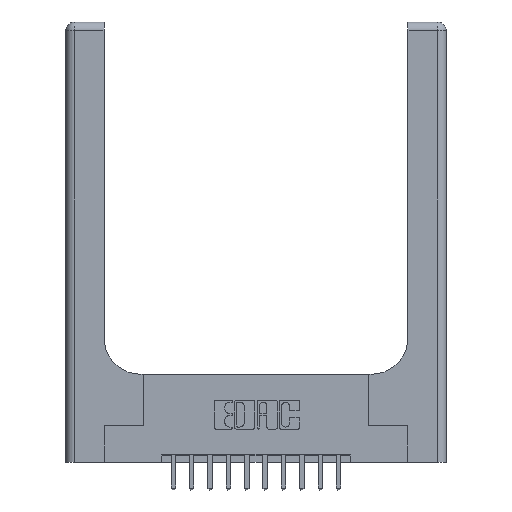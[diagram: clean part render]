
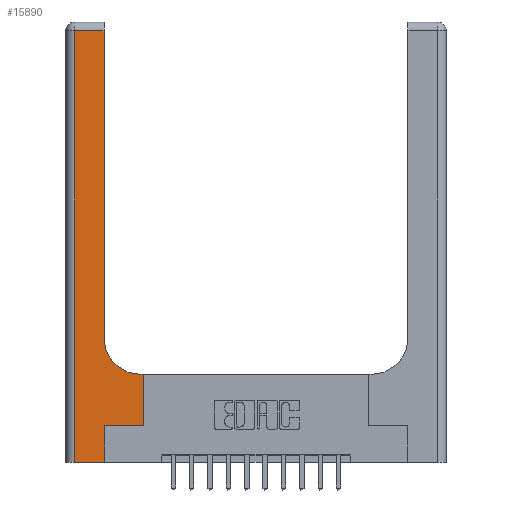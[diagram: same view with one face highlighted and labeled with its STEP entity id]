
A CAD part, top view. The second image highlights one B-rep face of the part: STEP entity #15890.
In plain terms, the highlighted planar face has unit normal (0, 0, 1).
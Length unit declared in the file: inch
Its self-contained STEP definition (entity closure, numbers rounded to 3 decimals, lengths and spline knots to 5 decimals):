
#78 = FACE_OUTER_BOUND ( 'NONE', #242, .T. ) ;
#242 = EDGE_LOOP ( 'NONE', ( #7406, #13943, #321, #14943, #8692, #8205, #9880, #706, #9428 ) ) ;
#321 = ORIENTED_EDGE ( 'NONE', *, *, #11762, .T. ) ;
#459 = LINE ( 'NONE', #12886, #14120 ) ;
#585 = DIRECTION ( 'NONE',  ( -1., 0., 0. ) ) ;
#706 = ORIENTED_EDGE ( 'NONE', *, *, #1168, .T. ) ;
#941 = CARTESIAN_POINT ( 'NONE',  ( 0., 2.94, 0.37 ) ) ;
#975 = DIRECTION ( 'NONE',  ( 0., 1., 0. ) ) ;
#1168 = EDGE_CURVE ( 'NONE', #1688, #16033, #459, .T. ) ;
#1455 = LINE ( 'NONE', #8380, #13540 ) ;
#1583 = LINE ( 'NONE', #3682, #7609 ) ;
#1688 = VERTEX_POINT ( 'NONE', #3864 ) ;
#1951 = VERTEX_POINT ( 'NONE', #8180 ) ;
#2025 = CARTESIAN_POINT ( 'NONE',  ( 0.265, 0.25, 0.37 ) ) ;
#2459 = LINE ( 'NONE', #13477, #3044 ) ;
#2479 = CARTESIAN_POINT ( 'NONE',  ( 0.06, 2.94, 0.37 ) ) ;
#2660 = CARTESIAN_POINT ( 'NONE',  ( 0.26, 2.94, 0.37 ) ) ;
#2893 = DIRECTION ( 'NONE',  ( 0., 0., -1. ) ) ;
#3044 = VECTOR ( 'NONE', #5995, 39.37008 ) ;
#3268 = VERTEX_POINT ( 'NONE', #5319 ) ;
#3651 = LINE ( 'NONE', #2025, #14383 ) ;
#3682 = CARTESIAN_POINT ( 'NONE',  ( 0., 0., 0.37 ) ) ;
#3766 = EDGE_CURVE ( 'NONE', #13320, #14780, #1583, .T. ) ;
#3864 = CARTESIAN_POINT ( 'NONE',  ( 0.528, 0.6, 0.37 ) ) ;
#4202 = AXIS2_PLACEMENT_3D ( 'NONE', #4292, #11835, #4339 ) ;
#4212 = LINE ( 'NONE', #8124, #10471 ) ;
#4292 = CARTESIAN_POINT ( 'NONE',  ( 0.51, 0.85, 0.37 ) ) ;
#4339 = DIRECTION ( 'NONE',  ( 1., 0., 0. ) ) ;
#4588 = VERTEX_POINT ( 'NONE', #2479 ) ;
#5138 = PLANE ( 'NONE',  #7584 ) ;
#5319 = CARTESIAN_POINT ( 'NONE',  ( 0.528, 0.25, 0.37 ) ) ;
#5873 = CARTESIAN_POINT ( 'NONE',  ( 0.26, 0.85, 0.37 ) ) ;
#5995 = DIRECTION ( 'NONE',  ( 0., 1., 0. ) ) ;
#6596 = DIRECTION ( 'NONE',  ( -1., 0., 0. ) ) ;
#6773 = EDGE_CURVE ( 'NONE', #3268, #1688, #4212, .T. ) ;
#6975 = DIRECTION ( 'NONE',  ( -1., 0., 0. ) ) ;
#7406 = ORIENTED_EDGE ( 'NONE', *, *, #7676, .T. ) ;
#7584 = AXIS2_PLACEMENT_3D ( 'NONE', #15113, #2893, #6596 ) ;
#7609 = VECTOR ( 'NONE', #14924, 39.37008 ) ;
#7676 = EDGE_CURVE ( 'NONE', #14758, #10249, #1455, .T. ) ;
#8124 = CARTESIAN_POINT ( 'NONE',  ( 0.528, 0.25, 0.37 ) ) ;
#8180 = CARTESIAN_POINT ( 'NONE',  ( 0.265, 0.25, 0.37 ) ) ;
#8205 = ORIENTED_EDGE ( 'NONE', *, *, #12205, .T. ) ;
#8338 = VECTOR ( 'NONE', #15241, 39.37008 ) ;
#8380 = CARTESIAN_POINT ( 'NONE',  ( 0.26, 3., 0.37 ) ) ;
#8692 = ORIENTED_EDGE ( 'NONE', *, *, #12348, .T. ) ;
#8872 = VECTOR ( 'NONE', #6975, 39.37008 ) ;
#9428 = ORIENTED_EDGE ( 'NONE', *, *, #9484, .T. ) ;
#9484 = EDGE_CURVE ( 'NONE', #16033, #14758, #10975, .T. ) ;
#9880 = ORIENTED_EDGE ( 'NONE', *, *, #6773, .T. ) ;
#10211 = CARTESIAN_POINT ( 'NONE',  ( 0.51, 0.6, 0.37 ) ) ;
#10249 = VERTEX_POINT ( 'NONE', #2660 ) ;
#10251 = CARTESIAN_POINT ( 'NONE',  ( 0.06, 3., 0.37 ) ) ;
#10471 = VECTOR ( 'NONE', #15707, 39.37008 ) ;
#10975 = CIRCLE ( 'NONE', #4202, 0.25 ) ;
#11762 = EDGE_CURVE ( 'NONE', #4588, #13320, #15170, .T. ) ;
#11835 = DIRECTION ( 'NONE',  ( 0., 0., -1. ) ) ;
#12204 = LINE ( 'NONE', #941, #8872 ) ;
#12205 = EDGE_CURVE ( 'NONE', #1951, #3268, #3651, .T. ) ;
#12348 = EDGE_CURVE ( 'NONE', #14780, #1951, #2459, .T. ) ;
#12701 = CARTESIAN_POINT ( 'NONE',  ( 0.06, 0., 0.37 ) ) ;
#12886 = CARTESIAN_POINT ( 'NONE',  ( 0.26, 0.6, 0.37 ) ) ;
#13320 = VERTEX_POINT ( 'NONE', #12701 ) ;
#13477 = CARTESIAN_POINT ( 'NONE',  ( 0.265, 0., 0.37 ) ) ;
#13540 = VECTOR ( 'NONE', #975, 39.37008 ) ;
#13943 = ORIENTED_EDGE ( 'NONE', *, *, #14156, .T. ) ;
#14120 = VECTOR ( 'NONE', #585, 39.37008 ) ;
#14156 = EDGE_CURVE ( 'NONE', #10249, #4588, #12204, .T. ) ;
#14383 = VECTOR ( 'NONE', #14410, 39.37008 ) ;
#14410 = DIRECTION ( 'NONE',  ( 1., 0., 0. ) ) ;
#14758 = VERTEX_POINT ( 'NONE', #5873 ) ;
#14780 = VERTEX_POINT ( 'NONE', #15873 ) ;
#14924 = DIRECTION ( 'NONE',  ( 1., 0., 0. ) ) ;
#14943 = ORIENTED_EDGE ( 'NONE', *, *, #3766, .T. ) ;
#15113 = CARTESIAN_POINT ( 'NONE',  ( 0., 3., 0.37 ) ) ;
#15170 = LINE ( 'NONE', #10251, #8338 ) ;
#15241 = DIRECTION ( 'NONE',  ( 0., -1., 0. ) ) ;
#15707 = DIRECTION ( 'NONE',  ( 0., 1., 0. ) ) ;
#15873 = CARTESIAN_POINT ( 'NONE',  ( 0.265, 0., 0.37 ) ) ;
#15890 = ADVANCED_FACE ( 'NONE', ( #78 ), #5138, .F. ) ;
#16033 = VERTEX_POINT ( 'NONE', #10211 ) ;
